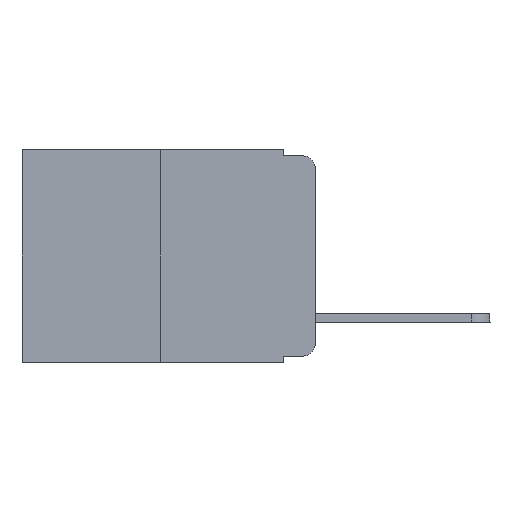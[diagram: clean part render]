
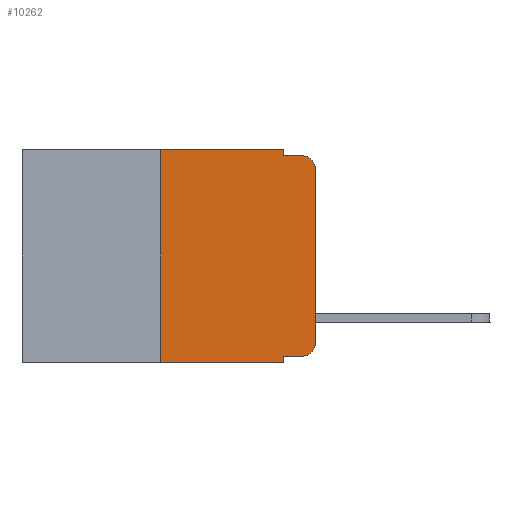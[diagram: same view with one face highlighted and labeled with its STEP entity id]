
A CAD part, left-side view. The second image highlights one B-rep face of the part: STEP entity #10262.
In plain terms, the highlighted planar face has unit normal (-1, 0, 0).
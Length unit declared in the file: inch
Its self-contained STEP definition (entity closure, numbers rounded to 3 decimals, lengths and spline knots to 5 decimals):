
#37 = DIRECTION ( 'NONE',  ( 0., -1., 0. ) ) ;
#68 = VERTEX_POINT ( 'NONE', #15686 ) ;
#222 = AXIS2_PLACEMENT_3D ( 'NONE', #14301, #18213, #3267 ) ;
#253 = ORIENTED_EDGE ( 'NONE', *, *, #10205, .F. ) ;
#1256 = EDGE_CURVE ( 'NONE', #6513, #14864, #13690, .T. ) ;
#1271 = ORIENTED_EDGE ( 'NONE', *, *, #12898, .T. ) ;
#1818 = EDGE_CURVE ( 'NONE', #7595, #5754, #1847, .T. ) ;
#1847 = LINE ( 'NONE', #19966, #23840 ) ;
#2032 = DIRECTION ( 'NONE',  ( 0., 0., -1. ) ) ;
#2147 = VERTEX_POINT ( 'NONE', #22676 ) ;
#2389 = VERTEX_POINT ( 'NONE', #8956 ) ;
#3131 = CARTESIAN_POINT ( 'NONE',  ( 0., 0.051, 0. ) ) ;
#3195 = EDGE_CURVE ( 'NONE', #13267, #19273, #22029, .T. ) ;
#3203 = CARTESIAN_POINT ( 'NONE',  ( 0., 0.02, -0.03 ) ) ;
#3267 = DIRECTION ( 'NONE',  ( 0., 0., -1. ) ) ;
#3325 = ORIENTED_EDGE ( 'NONE', *, *, #1256, .T. ) ;
#3454 = EDGE_CURVE ( 'NONE', #16462, #2389, #14758, .T. ) ;
#4406 = CARTESIAN_POINT ( 'NONE',  ( 0., 0.02, -0.313 ) ) ;
#5285 = LINE ( 'NONE', #9597, #18561 ) ;
#5441 = ORIENTED_EDGE ( 'NONE', *, *, #1818, .F. ) ;
#5754 = VERTEX_POINT ( 'NONE', #18217 ) ;
#5771 = DIRECTION ( 'NONE',  ( 0., 0., 1. ) ) ;
#6059 = DIRECTION ( 'NONE',  ( 0., 0., 1. ) ) ;
#6513 = VERTEX_POINT ( 'NONE', #22980 ) ;
#6891 = DIRECTION ( 'NONE',  ( 0., -1., 0. ) ) ;
#7201 = CARTESIAN_POINT ( 'NONE',  ( 0., 0.473, 0. ) ) ;
#7595 = VERTEX_POINT ( 'NONE', #3131 ) ;
#8678 = DIRECTION ( 'NONE',  ( 0., 0., -1. ) ) ;
#8705 = DIRECTION ( 'NONE',  ( -1., 0., 0. ) ) ;
#8956 = CARTESIAN_POINT ( 'NONE',  ( 0., 0., -0.313 ) ) ;
#9160 = DIRECTION ( 'NONE',  ( 0., -1., 0. ) ) ;
#9597 = CARTESIAN_POINT ( 'NONE',  ( 0., 0.051, -0.333 ) ) ;
#10205 = EDGE_CURVE ( 'NONE', #5754, #14864, #17791, .T. ) ;
#10262 = ADVANCED_FACE ( 'NONE', ( #13424 ), #12541, .F. ) ;
#11462 = CARTESIAN_POINT ( 'NONE',  ( 0., 0.051, -0.333 ) ) ;
#12201 = EDGE_CURVE ( 'NONE', #2147, #19273, #22630, .T. ) ;
#12286 = VECTOR ( 'NONE', #6891, 39.37008 ) ;
#12541 = PLANE ( 'NONE',  #222 ) ;
#12762 = EDGE_CURVE ( 'NONE', #68, #7595, #17394, .T. ) ;
#12898 = EDGE_CURVE ( 'NONE', #13267, #16462, #5285, .T. ) ;
#13080 = CARTESIAN_POINT ( 'NONE',  ( 0., 0., 0. ) ) ;
#13267 = VERTEX_POINT ( 'NONE', #11462 ) ;
#13424 = FACE_OUTER_BOUND ( 'NONE', #16434, .T. ) ;
#13547 = DIRECTION ( 'NONE',  ( -1., 0., 0. ) ) ;
#13627 = VECTOR ( 'NONE', #9160, 39.37008 ) ;
#13690 = CIRCLE ( 'NONE', #22216, 0.02 ) ;
#14301 = CARTESIAN_POINT ( 'NONE',  ( 0., 0.473, 0. ) ) ;
#14498 = LINE ( 'NONE', #13080, #17411 ) ;
#14758 = CIRCLE ( 'NONE', #18249, 0.02 ) ;
#14864 = VERTEX_POINT ( 'NONE', #17350 ) ;
#15033 = ORIENTED_EDGE ( 'NONE', *, *, #3195, .F. ) ;
#15205 = DIRECTION ( 'NONE',  ( 0., -1., 0. ) ) ;
#15596 = ORIENTED_EDGE ( 'NONE', *, *, #12201, .T. ) ;
#15686 = CARTESIAN_POINT ( 'NONE',  ( 0., 0.25, 0. ) ) ;
#16282 = LINE ( 'NONE', #18896, #17139 ) ;
#16434 = EDGE_LOOP ( 'NONE', ( #18614, #3325, #253, #5441, #17773, #21808, #15596, #15033, #1271, #23775 ) ) ;
#16462 = VERTEX_POINT ( 'NONE', #17193 ) ;
#17110 = VECTOR ( 'NONE', #2032, 39.37008 ) ;
#17139 = VECTOR ( 'NONE', #6059, 39.37008 ) ;
#17193 = CARTESIAN_POINT ( 'NONE',  ( 0., 0.02, -0.333 ) ) ;
#17350 = CARTESIAN_POINT ( 'NONE',  ( 0., 0.02, -0.01 ) ) ;
#17394 = LINE ( 'NONE', #7201, #13627 ) ;
#17411 = VECTOR ( 'NONE', #5771, 39.37008 ) ;
#17438 = VECTOR ( 'NONE', #37, 39.37008 ) ;
#17773 = ORIENTED_EDGE ( 'NONE', *, *, #12762, .F. ) ;
#17791 = LINE ( 'NONE', #21591, #12286 ) ;
#18213 = DIRECTION ( 'NONE',  ( 1., 0., 0. ) ) ;
#18217 = CARTESIAN_POINT ( 'NONE',  ( 0., 0.051, -0.01 ) ) ;
#18249 = AXIS2_PLACEMENT_3D ( 'NONE', #4406, #13547, #23112 ) ;
#18561 = VECTOR ( 'NONE', #15205, 39.37008 ) ;
#18614 = ORIENTED_EDGE ( 'NONE', *, *, #20913, .T. ) ;
#18896 = CARTESIAN_POINT ( 'NONE',  ( 0., 0.25, 0. ) ) ;
#19273 = VERTEX_POINT ( 'NONE', #21243 ) ;
#19966 = CARTESIAN_POINT ( 'NONE',  ( 0., 0.051, 0. ) ) ;
#20913 = EDGE_CURVE ( 'NONE', #2389, #6513, #14498, .T. ) ;
#21243 = CARTESIAN_POINT ( 'NONE',  ( 0., 0.051, -0.343 ) ) ;
#21591 = CARTESIAN_POINT ( 'NONE',  ( 0., 0.051, -0.01 ) ) ;
#21808 = ORIENTED_EDGE ( 'NONE', *, *, #23438, .F. ) ;
#22029 = LINE ( 'NONE', #22142, #17110 ) ;
#22142 = CARTESIAN_POINT ( 'NONE',  ( 0., 0.051, 0. ) ) ;
#22216 = AXIS2_PLACEMENT_3D ( 'NONE', #3203, #8705, #23487 ) ;
#22400 = CARTESIAN_POINT ( 'NONE',  ( 0., 0.473, -0.343 ) ) ;
#22630 = LINE ( 'NONE', #22400, #17438 ) ;
#22676 = CARTESIAN_POINT ( 'NONE',  ( 0., 0.25, -0.343 ) ) ;
#22980 = CARTESIAN_POINT ( 'NONE',  ( 0., 0., -0.03 ) ) ;
#23112 = DIRECTION ( 'NONE',  ( 0., 0., -1. ) ) ;
#23438 = EDGE_CURVE ( 'NONE', #2147, #68, #16282, .T. ) ;
#23487 = DIRECTION ( 'NONE',  ( 0., 0., -1. ) ) ;
#23775 = ORIENTED_EDGE ( 'NONE', *, *, #3454, .T. ) ;
#23840 = VECTOR ( 'NONE', #8678, 39.37008 ) ;
